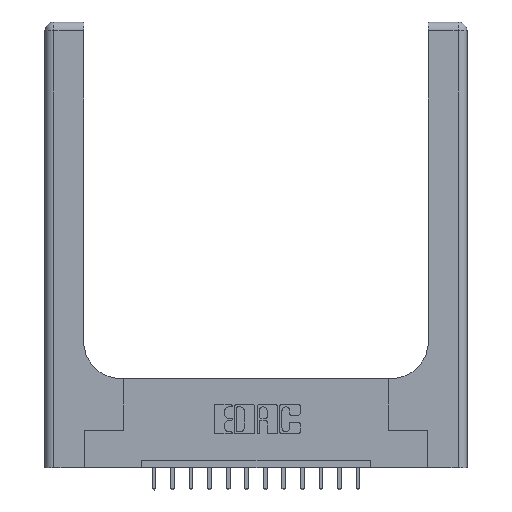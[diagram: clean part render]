
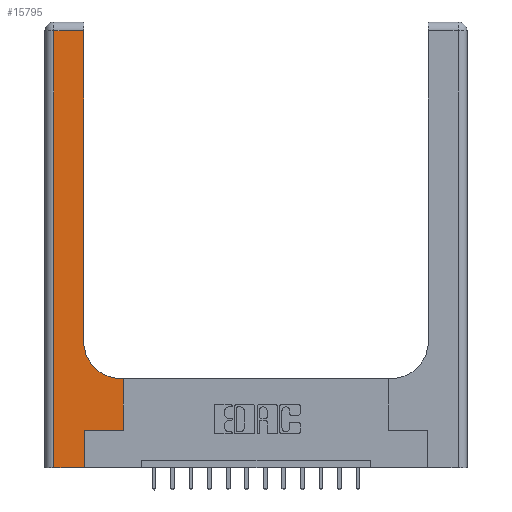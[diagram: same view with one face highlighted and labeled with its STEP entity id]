
A CAD part, top view. The second image highlights one B-rep face of the part: STEP entity #15795.
In plain terms, the highlighted planar face has unit normal (0, 0, 1).
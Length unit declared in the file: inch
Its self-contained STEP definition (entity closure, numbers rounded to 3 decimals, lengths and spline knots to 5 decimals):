
#251 = EDGE_CURVE ( 'NONE', #10598, #3073, #3948, .T. ) ;
#504 = CARTESIAN_POINT ( 'NONE',  ( 0., 2.94, 0.37 ) ) ;
#591 = LINE ( 'NONE', #6689, #2200 ) ;
#963 = LINE ( 'NONE', #504, #12108 ) ;
#1075 = VERTEX_POINT ( 'NONE', #8455 ) ;
#1380 = ORIENTED_EDGE ( 'NONE', *, *, #251, .T. ) ;
#1668 = ORIENTED_EDGE ( 'NONE', *, *, #14794, .T. ) ;
#1997 = ORIENTED_EDGE ( 'NONE', *, *, #3950, .T. ) ;
#2165 = ORIENTED_EDGE ( 'NONE', *, *, #14597, .T. ) ;
#2200 = VECTOR ( 'NONE', #10441, 39.37008 ) ;
#2347 = VERTEX_POINT ( 'NONE', #5052 ) ;
#2497 = VERTEX_POINT ( 'NONE', #12944 ) ;
#2633 = DIRECTION ( 'NONE',  ( 0., 1., 0. ) ) ;
#3012 = CARTESIAN_POINT ( 'NONE',  ( 0.51, 0.85, 0.37 ) ) ;
#3073 = VERTEX_POINT ( 'NONE', #11918 ) ;
#3074 = CARTESIAN_POINT ( 'NONE',  ( 0.26, 3., 0.37 ) ) ;
#3618 = ORIENTED_EDGE ( 'NONE', *, *, #13321, .T. ) ;
#3890 = EDGE_CURVE ( 'NONE', #1075, #10794, #591, .T. ) ;
#3948 = LINE ( 'NONE', #4444, #7988 ) ;
#3950 = EDGE_CURVE ( 'NONE', #10794, #13966, #5660, .T. ) ;
#4313 = DIRECTION ( 'NONE',  ( 0., 0., -1. ) ) ;
#4444 = CARTESIAN_POINT ( 'NONE',  ( 0., 0., 0.37 ) ) ;
#4835 = LINE ( 'NONE', #15455, #14745 ) ;
#5052 = CARTESIAN_POINT ( 'NONE',  ( 0.06, 2.94, 0.37 ) ) ;
#5132 = DIRECTION ( 'NONE',  ( 1., 0., 0. ) ) ;
#5436 = AXIS2_PLACEMENT_3D ( 'NONE', #11640, #10414, #6493 ) ;
#5443 = CARTESIAN_POINT ( 'NONE',  ( 0.528, 0.25, 0.37 ) ) ;
#5660 = CIRCLE ( 'NONE', #10389, 0.25 ) ;
#6034 = CARTESIAN_POINT ( 'NONE',  ( 0.528, 0.25, 0.37 ) ) ;
#6206 = VECTOR ( 'NONE', #13771, 39.37008 ) ;
#6493 = DIRECTION ( 'NONE',  ( -1., 0., 0. ) ) ;
#6527 = DIRECTION ( 'NONE',  ( 0., 1., 0. ) ) ;
#6689 = CARTESIAN_POINT ( 'NONE',  ( 0.26, 0.6, 0.37 ) ) ;
#6759 = VERTEX_POINT ( 'NONE', #7788 ) ;
#6788 = DIRECTION ( 'NONE',  ( 0., 1., 0. ) ) ;
#7106 = LINE ( 'NONE', #3074, #9554 ) ;
#7149 = DIRECTION ( 'NONE',  ( 1., 0., 0. ) ) ;
#7203 = VECTOR ( 'NONE', #6527, 39.37008 ) ;
#7262 = CARTESIAN_POINT ( 'NONE',  ( 0.06, 3., 0.37 ) ) ;
#7788 = CARTESIAN_POINT ( 'NONE',  ( 0.265, 0.25, 0.37 ) ) ;
#7988 = VECTOR ( 'NONE', #7149, 39.37008 ) ;
#8387 = ORIENTED_EDGE ( 'NONE', *, *, #11208, .T. ) ;
#8429 = CARTESIAN_POINT ( 'NONE',  ( 0.51, 0.6, 0.37 ) ) ;
#8455 = CARTESIAN_POINT ( 'NONE',  ( 0.528, 0.6, 0.37 ) ) ;
#8495 = ORIENTED_EDGE ( 'NONE', *, *, #15859, .T. ) ;
#8815 = LINE ( 'NONE', #5443, #7203 ) ;
#8987 = FACE_OUTER_BOUND ( 'NONE', #14607, .T. ) ;
#9022 = CARTESIAN_POINT ( 'NONE',  ( 0.265, 0.25, 0.37 ) ) ;
#9554 = VECTOR ( 'NONE', #6788, 39.37008 ) ;
#9713 = ORIENTED_EDGE ( 'NONE', *, *, #3890, .T. ) ;
#10362 = PLANE ( 'NONE',  #5436 ) ;
#10389 = AXIS2_PLACEMENT_3D ( 'NONE', #3012, #4313, #13340 ) ;
#10414 = DIRECTION ( 'NONE',  ( 0., 0., -1. ) ) ;
#10441 = DIRECTION ( 'NONE',  ( -1., 0., 0. ) ) ;
#10598 = VERTEX_POINT ( 'NONE', #15743 ) ;
#10636 = LINE ( 'NONE', #7262, #6206 ) ;
#10794 = VERTEX_POINT ( 'NONE', #8429 ) ;
#11208 = EDGE_CURVE ( 'NONE', #13966, #2497, #7106, .T. ) ;
#11640 = CARTESIAN_POINT ( 'NONE',  ( 0., 3., 0.37 ) ) ;
#11918 = CARTESIAN_POINT ( 'NONE',  ( 0.265, 0., 0.37 ) ) ;
#12108 = VECTOR ( 'NONE', #16039, 39.37008 ) ;
#12241 = VECTOR ( 'NONE', #5132, 39.37008 ) ;
#12855 = CARTESIAN_POINT ( 'NONE',  ( 0.26, 0.85, 0.37 ) ) ;
#12944 = CARTESIAN_POINT ( 'NONE',  ( 0.26, 2.94, 0.37 ) ) ;
#13219 = LINE ( 'NONE', #9022, #12241 ) ;
#13321 = EDGE_CURVE ( 'NONE', #3073, #6759, #4835, .T. ) ;
#13340 = DIRECTION ( 'NONE',  ( 1., 0., 0. ) ) ;
#13730 = EDGE_CURVE ( 'NONE', #2497, #2347, #963, .T. ) ;
#13771 = DIRECTION ( 'NONE',  ( 0., -1., 0. ) ) ;
#13966 = VERTEX_POINT ( 'NONE', #12855 ) ;
#14554 = VERTEX_POINT ( 'NONE', #6034 ) ;
#14597 = EDGE_CURVE ( 'NONE', #2347, #10598, #10636, .T. ) ;
#14607 = EDGE_LOOP ( 'NONE', ( #8387, #15918, #2165, #1380, #3618, #8495, #1668, #9713, #1997 ) ) ;
#14745 = VECTOR ( 'NONE', #2633, 39.37008 ) ;
#14794 = EDGE_CURVE ( 'NONE', #14554, #1075, #8815, .T. ) ;
#15455 = CARTESIAN_POINT ( 'NONE',  ( 0.265, 0., 0.37 ) ) ;
#15743 = CARTESIAN_POINT ( 'NONE',  ( 0.06, 0., 0.37 ) ) ;
#15795 = ADVANCED_FACE ( 'NONE', ( #8987 ), #10362, .F. ) ;
#15859 = EDGE_CURVE ( 'NONE', #6759, #14554, #13219, .T. ) ;
#15918 = ORIENTED_EDGE ( 'NONE', *, *, #13730, .T. ) ;
#16039 = DIRECTION ( 'NONE',  ( -1., 0., 0. ) ) ;
